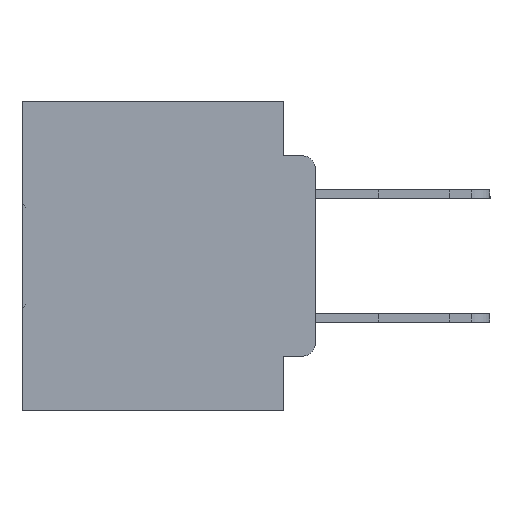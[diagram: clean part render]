
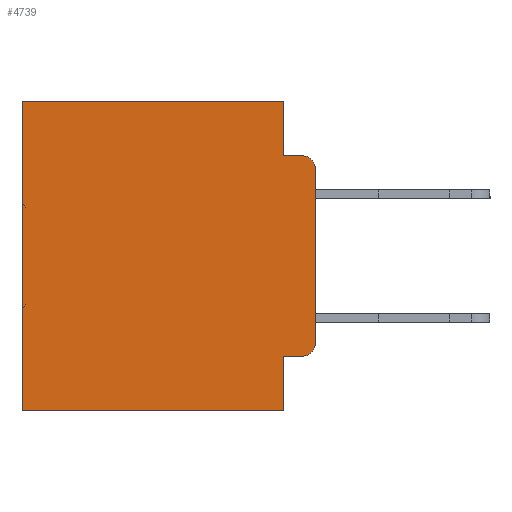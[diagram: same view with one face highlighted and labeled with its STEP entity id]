
A CAD part, left-side view. The second image highlights one B-rep face of the part: STEP entity #4739.
In plain terms, the highlighted planar face has unit normal (-1, 0, 0).
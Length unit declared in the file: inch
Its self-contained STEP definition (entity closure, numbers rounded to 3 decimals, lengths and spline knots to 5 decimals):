
#514 = VERTEX_POINT ( 'NONE', #21351 ) ;
#947 = CARTESIAN_POINT ( 'NONE',  ( 0.298, 0.473, 0. ) ) ;
#1010 = CARTESIAN_POINT ( 'NONE',  ( 0.298, 0.02, -0.0885 ) ) ;
#1747 = VECTOR ( 'NONE', #14401, 39.37008 ) ;
#1896 = CARTESIAN_POINT ( 'NONE',  ( 0.298, 0.051, -0.0885 ) ) ;
#1917 = AXIS2_PLACEMENT_3D ( 'NONE', #8337, #26887, #10979 ) ;
#2216 = VECTOR ( 'NONE', #24692, 39.37008 ) ;
#3002 = VECTOR ( 'NONE', #33923, 39.37008 ) ;
#3845 = LINE ( 'NONE', #18125, #3002 ) ;
#4070 = VERTEX_POINT ( 'NONE', #12393 ) ;
#4295 = VERTEX_POINT ( 'NONE', #8688 ) ;
#4739 = ADVANCED_FACE ( 'NONE', ( #9021 ), #27486, .F. ) ;
#5123 = DIRECTION ( 'NONE',  ( 0., 0., -1. ) ) ;
#5377 = CARTESIAN_POINT ( 'NONE',  ( 0.298, 0.473, -0.5 ) ) ;
#6222 = ORIENTED_EDGE ( 'NONE', *, *, #7422, .F. ) ;
#6276 = ORIENTED_EDGE ( 'NONE', *, *, #27637, .F. ) ;
#6702 = CARTESIAN_POINT ( 'NONE',  ( 0.298, 0., 0. ) ) ;
#7422 = EDGE_CURVE ( 'NONE', #14337, #22763, #23409, .T. ) ;
#7472 = DIRECTION ( 'NONE',  ( -1., 0., 0. ) ) ;
#7978 = CIRCLE ( 'NONE', #1917, 0.02 ) ;
#8120 = CARTESIAN_POINT ( 'NONE',  ( 0.298, 0., -0.5 ) ) ;
#8337 = CARTESIAN_POINT ( 'NONE',  ( 0.298, 0.02, -0.3915 ) ) ;
#8688 = CARTESIAN_POINT ( 'NONE',  ( 0.298, 0.02, -0.4115 ) ) ;
#8802 = ORIENTED_EDGE ( 'NONE', *, *, #32914, .T. ) ;
#9021 = FACE_OUTER_BOUND ( 'NONE', #25853, .T. ) ;
#9326 = VECTOR ( 'NONE', #14591, 39.37008 ) ;
#9760 = CARTESIAN_POINT ( 'NONE',  ( 0.298, 0.051, -0.4115 ) ) ;
#10527 = VERTEX_POINT ( 'NONE', #5377 ) ;
#10946 = EDGE_CURVE ( 'NONE', #4070, #10527, #12046, .T. ) ;
#10979 = DIRECTION ( 'NONE',  ( 0., 0., -1. ) ) ;
#12020 = VECTOR ( 'NONE', #17841, 39.37008 ) ;
#12046 = LINE ( 'NONE', #947, #19953 ) ;
#12393 = CARTESIAN_POINT ( 'NONE',  ( 0.298, 0.473, 0. ) ) ;
#14086 = LINE ( 'NONE', #8120, #28174 ) ;
#14224 = AXIS2_PLACEMENT_3D ( 'NONE', #23343, #7472, #26019 ) ;
#14337 = VERTEX_POINT ( 'NONE', #9760 ) ;
#14401 = DIRECTION ( 'NONE',  ( 0., 0., -1. ) ) ;
#14443 = CARTESIAN_POINT ( 'NONE',  ( 0.298, 0.051, -0.5 ) ) ;
#14591 = DIRECTION ( 'NONE',  ( 0., -1., 0. ) ) ;
#14649 = VERTEX_POINT ( 'NONE', #29709 ) ;
#15577 = LINE ( 'NONE', #17258, #9326 ) ;
#16315 = EDGE_CURVE ( 'NONE', #29325, #19337, #3845, .T. ) ;
#17258 = CARTESIAN_POINT ( 'NONE',  ( 0.298, 0.051, -0.4115 ) ) ;
#17415 = EDGE_CURVE ( 'NONE', #29325, #4070, #32930, .T. ) ;
#17841 = DIRECTION ( 'NONE',  ( 0., -1., 0. ) ) ;
#18125 = CARTESIAN_POINT ( 'NONE',  ( 0.298, 0.051, 0. ) ) ;
#19119 = ORIENTED_EDGE ( 'NONE', *, *, #17415, .T. ) ;
#19337 = VERTEX_POINT ( 'NONE', #23161 ) ;
#19433 = DIRECTION ( 'NONE',  ( 0., 0., -1. ) ) ;
#19848 = EDGE_CURVE ( 'NONE', #19337, #25375, #20774, .T. ) ;
#19953 = VECTOR ( 'NONE', #19433, 39.37008 ) ;
#20774 = LINE ( 'NONE', #1896, #12020 ) ;
#21257 = ORIENTED_EDGE ( 'NONE', *, *, #16315, .F. ) ;
#21351 = CARTESIAN_POINT ( 'NONE',  ( 0.298, 0., -0.1085 ) ) ;
#21557 = CIRCLE ( 'NONE', #14224, 0.02 ) ;
#22695 = DIRECTION ( 'NONE',  ( 0., 1., 0. ) ) ;
#22763 = VERTEX_POINT ( 'NONE', #14443 ) ;
#22943 = LINE ( 'NONE', #30299, #1747 ) ;
#23161 = CARTESIAN_POINT ( 'NONE',  ( 0.298, 0.051, -0.0885 ) ) ;
#23343 = CARTESIAN_POINT ( 'NONE',  ( 0.298, 0.02, -0.1085 ) ) ;
#23409 = LINE ( 'NONE', #24408, #2216 ) ;
#23690 = ORIENTED_EDGE ( 'NONE', *, *, #19848, .F. ) ;
#23738 = AXIS2_PLACEMENT_3D ( 'NONE', #6702, #31570, #5123 ) ;
#24408 = CARTESIAN_POINT ( 'NONE',  ( 0.298, 0.051, 0. ) ) ;
#24692 = DIRECTION ( 'NONE',  ( 0., 0., -1. ) ) ;
#24990 = ORIENTED_EDGE ( 'NONE', *, *, #25868, .T. ) ;
#25375 = VERTEX_POINT ( 'NONE', #1010 ) ;
#25853 = EDGE_LOOP ( 'NONE', ( #30193, #28504, #23690, #21257, #19119, #27070, #6276, #6222, #8802, #24990 ) ) ;
#25868 = EDGE_CURVE ( 'NONE', #4295, #14649, #7978, .T. ) ;
#26019 = DIRECTION ( 'NONE',  ( 0., 0., -1. ) ) ;
#26100 = CARTESIAN_POINT ( 'NONE',  ( 0.298, 0.051, 0. ) ) ;
#26683 = DIRECTION ( 'NONE',  ( 0., 1., 0. ) ) ;
#26764 = VECTOR ( 'NONE', #22695, 39.37008 ) ;
#26887 = DIRECTION ( 'NONE',  ( -1., 0., 0. ) ) ;
#26967 = EDGE_CURVE ( 'NONE', #514, #25375, #21557, .T. ) ;
#27070 = ORIENTED_EDGE ( 'NONE', *, *, #10946, .T. ) ;
#27486 = PLANE ( 'NONE',  #23738 ) ;
#27637 = EDGE_CURVE ( 'NONE', #22763, #10527, #14086, .T. ) ;
#28035 = CARTESIAN_POINT ( 'NONE',  ( 0.298, 0., 0. ) ) ;
#28174 = VECTOR ( 'NONE', #26683, 39.37008 ) ;
#28504 = ORIENTED_EDGE ( 'NONE', *, *, #26967, .T. ) ;
#29325 = VERTEX_POINT ( 'NONE', #26100 ) ;
#29709 = CARTESIAN_POINT ( 'NONE',  ( 0.298, 0., -0.3915 ) ) ;
#30193 = ORIENTED_EDGE ( 'NONE', *, *, #34017, .F. ) ;
#30299 = CARTESIAN_POINT ( 'NONE',  ( 0.298, 0., 0. ) ) ;
#31570 = DIRECTION ( 'NONE',  ( 1., 0., 0. ) ) ;
#32914 = EDGE_CURVE ( 'NONE', #14337, #4295, #15577, .T. ) ;
#32930 = LINE ( 'NONE', #28035, #26764 ) ;
#33923 = DIRECTION ( 'NONE',  ( 0., 0., -1. ) ) ;
#34017 = EDGE_CURVE ( 'NONE', #514, #14649, #22943, .T. ) ;
